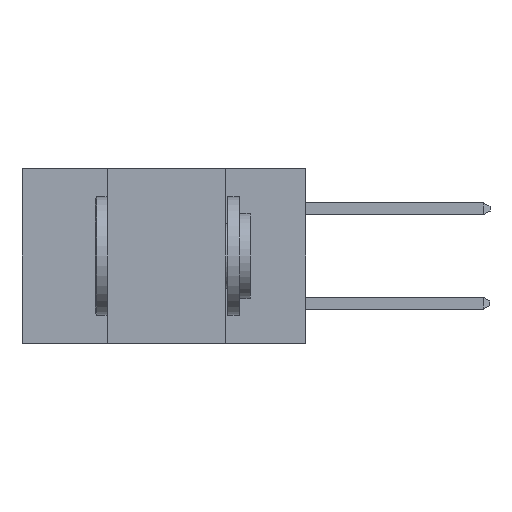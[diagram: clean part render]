
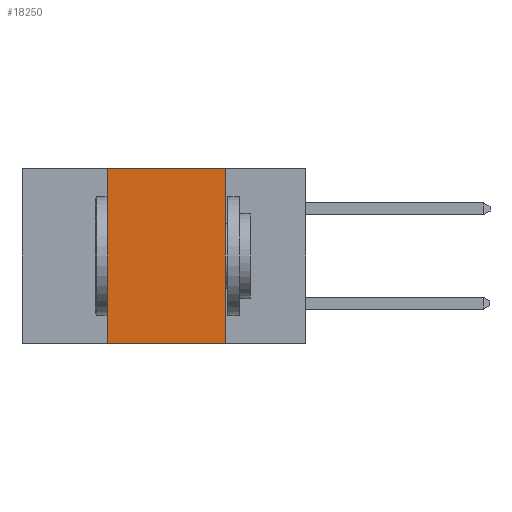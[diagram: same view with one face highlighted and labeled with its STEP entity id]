
A CAD part, left-side view. The second image highlights one B-rep face of the part: STEP entity #18250.
In plain terms, the highlighted planar face has unit normal (-1, 0, 0).
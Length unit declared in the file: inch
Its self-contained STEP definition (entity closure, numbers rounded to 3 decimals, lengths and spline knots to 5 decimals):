
#483 = EDGE_CURVE ( 'NONE', #11105, #8205, #6254, .T. ) ;
#1248 = VECTOR ( 'NONE', #22315, 39.37008 ) ;
#1276 = DIRECTION ( 'NONE',  ( 1., 0., 0. ) ) ;
#1905 = VERTEX_POINT ( 'NONE', #11019 ) ;
#2252 = DIRECTION ( 'NONE',  ( 0., -1., 0. ) ) ;
#2336 = LINE ( 'NONE', #22679, #20581 ) ;
#2435 = LINE ( 'NONE', #13562, #6879 ) ;
#3236 = FACE_OUTER_BOUND ( 'NONE', #19905, .T. ) ;
#4074 = ORIENTED_EDGE ( 'NONE', *, *, #5492, .F. ) ;
#4299 = CARTESIAN_POINT ( 'NONE',  ( 0., 0.17, 0. ) ) ;
#4654 = ORIENTED_EDGE ( 'NONE', *, *, #13878, .F. ) ;
#4929 = PLANE ( 'NONE',  #21595 ) ;
#4932 = ORIENTED_EDGE ( 'NONE', *, *, #483, .T. ) ;
#5492 = EDGE_CURVE ( 'NONE', #1905, #20054, #2435, .T. ) ;
#5886 = DIRECTION ( 'NONE',  ( 0., 0., 1. ) ) ;
#6238 = DIRECTION ( 'NONE',  ( 0., 0., -1. ) ) ;
#6254 = LINE ( 'NONE', #9723, #1248 ) ;
#6879 = VECTOR ( 'NONE', #2252, 39.37008 ) ;
#8205 = VERTEX_POINT ( 'NONE', #20882 ) ;
#9723 = CARTESIAN_POINT ( 'NONE',  ( 0., 0.6, -0.37 ) ) ;
#11019 = CARTESIAN_POINT ( 'NONE',  ( 0., 0.42, 0. ) ) ;
#11105 = VERTEX_POINT ( 'NONE', #21261 ) ;
#12371 = EDGE_CURVE ( 'NONE', #11105, #1905, #2336, .T. ) ;
#12584 = CARTESIAN_POINT ( 'NONE',  ( 0., 0.6, 0. ) ) ;
#13562 = CARTESIAN_POINT ( 'NONE',  ( 0., 0.6, 0. ) ) ;
#13878 = EDGE_CURVE ( 'NONE', #20054, #8205, #21361, .T. ) ;
#14466 = DIRECTION ( 'NONE',  ( 0., 0., -1. ) ) ;
#16202 = CARTESIAN_POINT ( 'NONE',  ( 0., 0.17, 0. ) ) ;
#16436 = VECTOR ( 'NONE', #6238, 39.37008 ) ;
#16821 = ORIENTED_EDGE ( 'NONE', *, *, #12371, .F. ) ;
#18250 = ADVANCED_FACE ( 'NONE', ( #3236 ), #4929, .F. ) ;
#19905 = EDGE_LOOP ( 'NONE', ( #4654, #4074, #16821, #4932 ) ) ;
#20054 = VERTEX_POINT ( 'NONE', #16202 ) ;
#20581 = VECTOR ( 'NONE', #5886, 39.37008 ) ;
#20882 = CARTESIAN_POINT ( 'NONE',  ( 0., 0.17, -0.37 ) ) ;
#21261 = CARTESIAN_POINT ( 'NONE',  ( 0., 0.42, -0.37 ) ) ;
#21361 = LINE ( 'NONE', #4299, #16436 ) ;
#21595 = AXIS2_PLACEMENT_3D ( 'NONE', #12584, #1276, #14466 ) ;
#22315 = DIRECTION ( 'NONE',  ( 0., -1., 0. ) ) ;
#22679 = CARTESIAN_POINT ( 'NONE',  ( 0., 0.42, 0. ) ) ;
